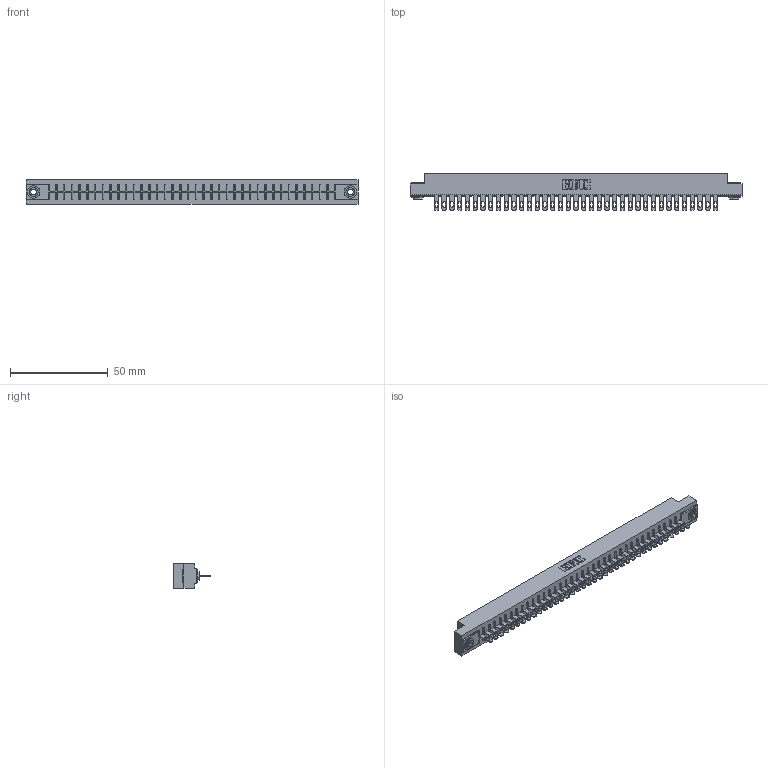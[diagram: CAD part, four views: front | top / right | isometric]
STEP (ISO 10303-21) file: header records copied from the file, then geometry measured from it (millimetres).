
FILE_DESCRIPTION (( 'STEP AP203' ), '1' );
FILE_NAME ('306-037-400-103.STEP', '2020-09-22T04:47:20', ( '' ), ( '' ), 'SwSTEP 2.0', 'SolidWorks 2020', '' );
FILE_SCHEMA (( 'CONFIG_CONTROL_DESIGN' ));
Length unit declared in the file: inch
Products named in the file (4): 306 Part_.156 Dia; 345-250-002_345-250-002-102; 306-290-001_100; 306-037-400-103
Assembly tree (40 placements, depth 2):
  306-037-400-103
    306 Part_.156 Dia
    306-290-001_100  x37
    345-250-002_345-250-002-102  x2
Bounding box: 169.62 x 18.87 x 12.7 mm (x, y, z)
Volume: 18831.9 mm3; surface area: 20184.7 mm2
Topology: 40 solids, 40 shells, 2980 faces, 8383 edges, 5386 vertices
Faces by surface type: plane 1942, cylinder 882, sphere 148, cone 8
Entity records: 36381 total; most frequent: CARTESIAN_POINT 6087, ORIENTED_EDGE 6026, DIRECTION 6017, EDGE_CURVE 3013, VECTOR 2345, LINE 2345, VERTEX_POINT 1906, AXIS2_PLACEMENT_3D 1836
